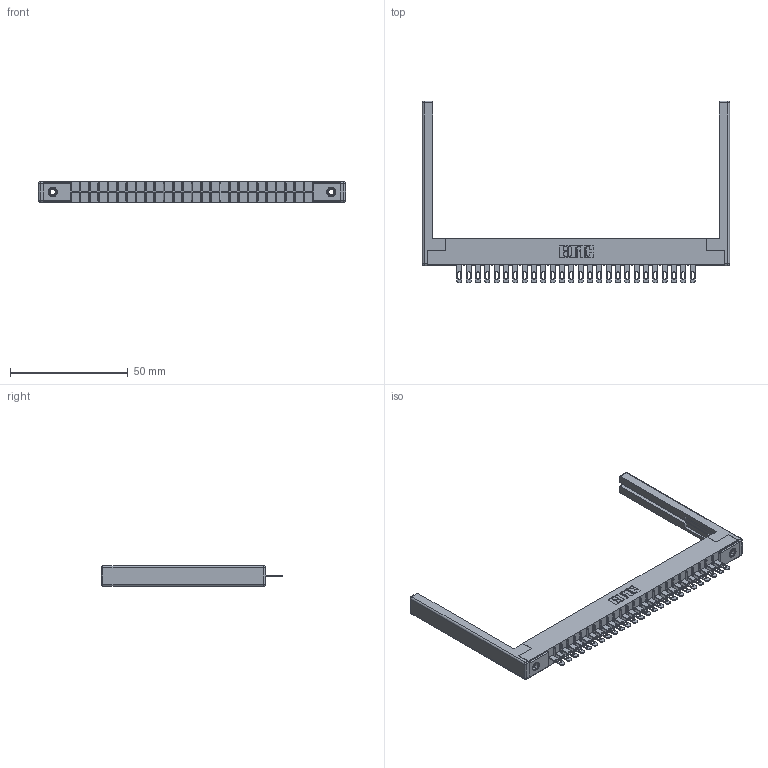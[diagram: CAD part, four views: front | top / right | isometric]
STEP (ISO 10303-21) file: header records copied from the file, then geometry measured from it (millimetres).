
FILE_DESCRIPTION (( 'STEP AP203' ), '1' );
FILE_NAME ('306-026-400-168.STEP', '2020-09-21T23:06:59', ( '' ), ( '' ), 'SwSTEP 2.0', 'SolidWorks 2020', '' );
FILE_SCHEMA (( 'CONFIG_CONTROL_DESIGN' ));
Length unit declared in the file: inch
Products named in the file (5): 306-026-400-168; 306 Part_.156 Dia; 345-250-001_345-250-001-102; 306-290-001_100; 307-220-068
Assembly tree (31 placements, depth 2):
  306-026-400-168
    306 Part_.156 Dia
    306-290-001_100  x26
    345-250-001_345-250-001-102  x2
    307-220-068  x2
Bounding box: 130.45 x 77.17 x 8.71 mm (x, y, z)
Volume: 13567.6 mm3; surface area: 17996.8 mm2
Topology: 31 solids, 31 shells, 2246 faces, 6296 edges, 4036 vertices
Faces by surface type: plane 1456, cylinder 662, sphere 112, cone 12, torus 4
Entity records: 29242 total; most frequent: CARTESIAN_POINT 4874, ORIENTED_EDGE 4822, DIRECTION 4821, EDGE_CURVE 2411, VECTOR 1871, LINE 1871, VERTEX_POINT 1528, AXIS2_PLACEMENT_3D 1475
